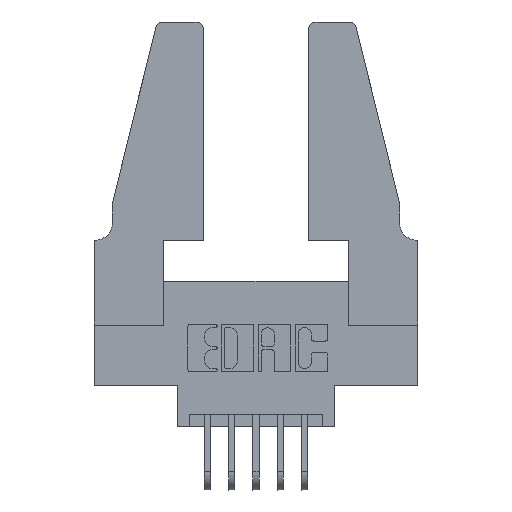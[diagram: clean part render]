
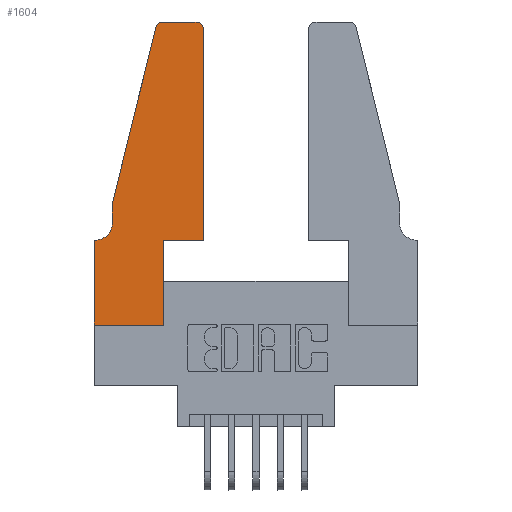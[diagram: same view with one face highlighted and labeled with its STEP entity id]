
A CAD part, top view. The second image highlights one B-rep face of the part: STEP entity #1604.
In plain terms, the highlighted planar face has unit normal (0, 0, 1).
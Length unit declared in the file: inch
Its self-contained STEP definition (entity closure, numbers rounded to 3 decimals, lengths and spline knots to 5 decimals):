
#27 = ORIENTED_EDGE ( 'NONE', *, *, #8061, .T. ) ;
#64 = DIRECTION ( 'NONE',  ( 0., -1., 0. ) ) ;
#107 = FACE_OUTER_BOUND ( 'NONE', #12073, .T. ) ;
#119 = DIRECTION ( 'NONE',  ( 1., 0., 0. ) ) ;
#372 = DIRECTION ( 'NONE',  ( 1., 0., 0. ) ) ;
#545 = EDGE_CURVE ( 'NONE', #4743, #2948, #9323, .T. ) ;
#740 = ORIENTED_EDGE ( 'NONE', *, *, #3014, .T. ) ;
#838 = CARTESIAN_POINT ( 'NONE',  ( 0.2865, 0.35, 0.37 ) ) ;
#1003 = VERTEX_POINT ( 'NONE', #12529 ) ;
#1347 = ORIENTED_EDGE ( 'NONE', *, *, #8027, .T. ) ;
#1439 = AXIS2_PLACEMENT_3D ( 'NONE', #3019, #11921, #9739 ) ;
#1520 = CARTESIAN_POINT ( 'NONE',  ( 0.0055, 0.42, 0.37 ) ) ;
#1532 = ORIENTED_EDGE ( 'NONE', *, *, #8240, .T. ) ;
#1604 = ADVANCED_FACE ( 'NONE', ( #107 ), #10724, .T. ) ;
#1751 = EDGE_CURVE ( 'NONE', #7112, #10867, #10664, .T. ) ;
#1789 = VECTOR ( 'NONE', #64, 39.37008 ) ;
#2352 = CARTESIAN_POINT ( 'NONE',  ( 0.2605, 1.25, 0.37 ) ) ;
#2611 = LINE ( 'NONE', #838, #7874 ) ;
#2866 = DIRECTION ( 'NONE',  ( -1., 0., 0. ) ) ;
#2948 = VERTEX_POINT ( 'NONE', #11167 ) ;
#2959 = DIRECTION ( 'NONE',  ( 0., 1., 0. ) ) ;
#3014 = EDGE_CURVE ( 'NONE', #2948, #3870, #4585, .T. ) ;
#3019 = CARTESIAN_POINT ( 'NONE',  ( 0.4205, 1.22, 0.37 ) ) ;
#3097 = ORIENTED_EDGE ( 'NONE', *, *, #7943, .T. ) ;
#3220 = VERTEX_POINT ( 'NONE', #9836 ) ;
#3426 = EDGE_CURVE ( 'NONE', #10673, #6543, #5820, .T. ) ;
#3755 = ORIENTED_EDGE ( 'NONE', *, *, #545, .T. ) ;
#3870 = VERTEX_POINT ( 'NONE', #5290 ) ;
#4585 = CIRCLE ( 'NONE', #1439, 0.03 ) ;
#4683 = DIRECTION ( 'NONE',  ( 1., 0., 0. ) ) ;
#4728 = ORIENTED_EDGE ( 'NONE', *, *, #1751, .T. ) ;
#4743 = VERTEX_POINT ( 'NONE', #9322 ) ;
#4996 = VERTEX_POINT ( 'NONE', #11810 ) ;
#5037 = ORIENTED_EDGE ( 'NONE', *, *, #5152, .T. ) ;
#5152 = EDGE_CURVE ( 'NONE', #12076, #3220, #10589, .T. ) ;
#5290 = CARTESIAN_POINT ( 'NONE',  ( 0.4205, 1.25, 0.37 ) ) ;
#5331 = LINE ( 'NONE', #12077, #1789 ) ;
#5371 = LINE ( 'NONE', #11449, #10331 ) ;
#5507 = VECTOR ( 'NONE', #4683, 39.37008 ) ;
#5707 = CARTESIAN_POINT ( 'NONE',  ( 0.0755, 0.5, 0.37 ) ) ;
#5807 = DIRECTION ( 'NONE',  ( -1., 0., 0. ) ) ;
#5814 = VERTEX_POINT ( 'NONE', #9399 ) ;
#5820 = LINE ( 'NONE', #10628, #5507 ) ;
#5946 = EDGE_CURVE ( 'NONE', #3220, #1003, #10399, .T. ) ;
#6271 = DIRECTION ( 'NONE',  ( -1., 0., 0. ) ) ;
#6412 = CARTESIAN_POINT ( 'NONE',  ( 0., 0., 0.37 ) ) ;
#6543 = VERTEX_POINT ( 'NONE', #7516 ) ;
#6765 = ORIENTED_EDGE ( 'NONE', *, *, #6787, .T. ) ;
#6787 = EDGE_CURVE ( 'NONE', #3870, #7112, #12731, .T. ) ;
#6794 = DIRECTION ( 'NONE',  ( 0., -1., 0. ) ) ;
#6833 = DIRECTION ( 'NONE',  ( 0., 1., 0. ) ) ;
#6874 = CARTESIAN_POINT ( 'NONE',  ( 0.4505, 0.35, 0.37 ) ) ;
#7088 = AXIS2_PLACEMENT_3D ( 'NONE', #8000, #8084, #119 ) ;
#7112 = VERTEX_POINT ( 'NONE', #11655 ) ;
#7164 = ORIENTED_EDGE ( 'NONE', *, *, #9261, .T. ) ;
#7298 = CARTESIAN_POINT ( 'NONE',  ( 0.25487, 1.22718, 0.37 ) ) ;
#7330 = VECTOR ( 'NONE', #6833, 39.37008 ) ;
#7356 = CARTESIAN_POINT ( 'NONE',  ( 0.0755, 0.42, 0.37 ) ) ;
#7516 = CARTESIAN_POINT ( 'NONE',  ( 0.2865, 0., 0.37 ) ) ;
#7813 = DIRECTION ( 'NONE',  ( 0., 0., 1. ) ) ;
#7874 = VECTOR ( 'NONE', #2959, 39.37008 ) ;
#7943 = EDGE_CURVE ( 'NONE', #10867, #4996, #9376, .T. ) ;
#8000 = CARTESIAN_POINT ( 'NONE',  ( 0.284, 1.22, 0.37 ) ) ;
#8027 = EDGE_CURVE ( 'NONE', #6543, #5814, #2611, .T. ) ;
#8061 = EDGE_CURVE ( 'NONE', #1003, #10673, #12215, .T. ) ;
#8084 = DIRECTION ( 'NONE',  ( 0., 0., 1. ) ) ;
#8204 = VECTOR ( 'NONE', #2866, 39.37008 ) ;
#8240 = EDGE_CURVE ( 'NONE', #5814, #4743, #5371, .T. ) ;
#8648 = AXIS2_PLACEMENT_3D ( 'NONE', #9952, #7813, #9996 ) ;
#8755 = CARTESIAN_POINT ( 'NONE',  ( 0.0755, 0.35, 0.37 ) ) ;
#9261 = EDGE_CURVE ( 'NONE', #4996, #12076, #5331, .T. ) ;
#9322 = CARTESIAN_POINT ( 'NONE',  ( 0.4505, 0.35, 0.37 ) ) ;
#9323 = LINE ( 'NONE', #6874, #7330 ) ;
#9376 = LINE ( 'NONE', #5707, #10963 ) ;
#9399 = CARTESIAN_POINT ( 'NONE',  ( 0.2865, 0.35, 0.37 ) ) ;
#9705 = VECTOR ( 'NONE', #6794, 39.37008 ) ;
#9739 = DIRECTION ( 'NONE',  ( 1., 0., 0. ) ) ;
#9836 = CARTESIAN_POINT ( 'NONE',  ( 0.0055, 0.35, 0.37 ) ) ;
#9952 = CARTESIAN_POINT ( 'NONE',  ( 0., 0.35, 0.37 ) ) ;
#9996 = DIRECTION ( 'NONE',  ( 1., 0., 0. ) ) ;
#10063 = ORIENTED_EDGE ( 'NONE', *, *, #5946, .T. ) ;
#10331 = VECTOR ( 'NONE', #372, 39.37008 ) ;
#10399 = LINE ( 'NONE', #8755, #8204 ) ;
#10539 = VECTOR ( 'NONE', #6271, 39.37008 ) ;
#10589 = CIRCLE ( 'NONE', #11255, 0.07 ) ;
#10628 = CARTESIAN_POINT ( 'NONE',  ( 0., 0., 0.37 ) ) ;
#10664 = CIRCLE ( 'NONE', #7088, 0.03 ) ;
#10673 = VERTEX_POINT ( 'NONE', #6412 ) ;
#10724 = PLANE ( 'NONE',  #8648 ) ;
#10867 = VERTEX_POINT ( 'NONE', #7298 ) ;
#10963 = VECTOR ( 'NONE', #12660, 39.37008 ) ;
#11167 = CARTESIAN_POINT ( 'NONE',  ( 0.4505, 1.22, 0.37 ) ) ;
#11255 = AXIS2_PLACEMENT_3D ( 'NONE', #1520, #11457, #5807 ) ;
#11449 = CARTESIAN_POINT ( 'NONE',  ( 0.4505, 0.35, 0.37 ) ) ;
#11457 = DIRECTION ( 'NONE',  ( 0., 0., -1. ) ) ;
#11520 = ORIENTED_EDGE ( 'NONE', *, *, #3426, .T. ) ;
#11655 = CARTESIAN_POINT ( 'NONE',  ( 0.284, 1.25, 0.37 ) ) ;
#11810 = CARTESIAN_POINT ( 'NONE',  ( 0.0755, 0.5, 0.37 ) ) ;
#11921 = DIRECTION ( 'NONE',  ( 0., 0., 1. ) ) ;
#12073 = EDGE_LOOP ( 'NONE', ( #6765, #4728, #3097, #7164, #5037, #10063, #27, #11520, #1347, #1532, #3755, #740 ) ) ;
#12076 = VERTEX_POINT ( 'NONE', #7356 ) ;
#12077 = CARTESIAN_POINT ( 'NONE',  ( 0.0755, 0.5, 0.37 ) ) ;
#12215 = LINE ( 'NONE', #12749, #9705 ) ;
#12529 = CARTESIAN_POINT ( 'NONE',  ( 0., 0.35, 0.37 ) ) ;
#12660 = DIRECTION ( 'NONE',  ( -0.239, -0.971, 0. ) ) ;
#12731 = LINE ( 'NONE', #2352, #10539 ) ;
#12749 = CARTESIAN_POINT ( 'NONE',  ( 0., 0., 0.37 ) ) ;
